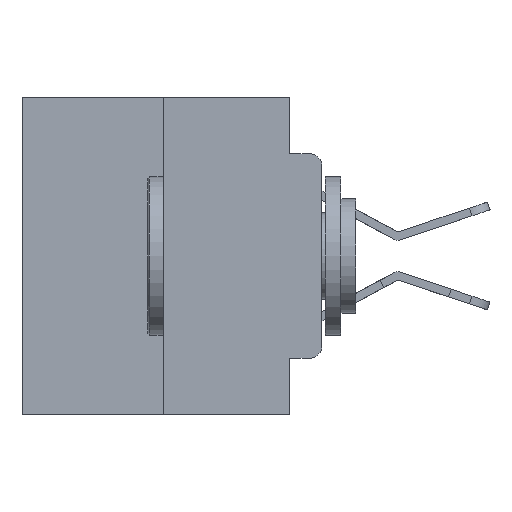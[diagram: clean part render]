
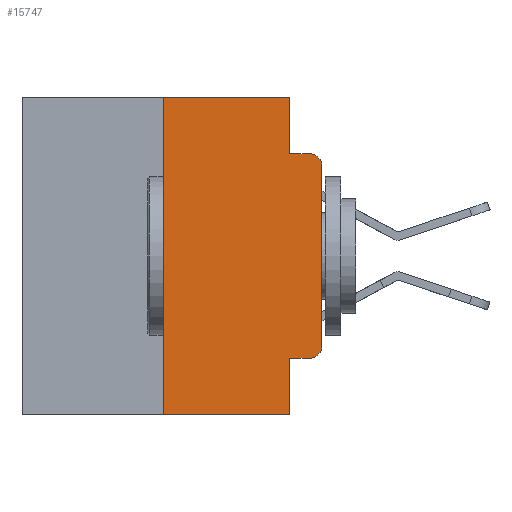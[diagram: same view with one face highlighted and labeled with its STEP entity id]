
A CAD part, left-side view. The second image highlights one B-rep face of the part: STEP entity #15747.
In plain terms, the highlighted planar face has unit normal (-1, 0, 0).
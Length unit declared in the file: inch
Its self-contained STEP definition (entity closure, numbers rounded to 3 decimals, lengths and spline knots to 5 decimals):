
#317 = VECTOR ( 'NONE', #20871, 39.37008 ) ;
#579 = LINE ( 'NONE', #9387, #16527 ) ;
#1281 = CARTESIAN_POINT ( 'NONE',  ( 0., 0.051, -0.5 ) ) ;
#1337 = AXIS2_PLACEMENT_3D ( 'NONE', #26024, #19266, #27897 ) ;
#2168 = CARTESIAN_POINT ( 'NONE',  ( 0., 0.473, 0. ) ) ;
#2622 = EDGE_CURVE ( 'NONE', #16160, #18057, #3386, .T. ) ;
#3017 = LINE ( 'NONE', #12999, #14215 ) ;
#3018 = LINE ( 'NONE', #6494, #4365 ) ;
#3276 = CARTESIAN_POINT ( 'NONE',  ( 0., 0., -0.1085 ) ) ;
#3386 = CIRCLE ( 'NONE', #24783, 0.02 ) ;
#3666 = ORIENTED_EDGE ( 'NONE', *, *, #14848, .F. ) ;
#4170 = DIRECTION ( 'NONE',  ( 0., 0., 1. ) ) ;
#4365 = VECTOR ( 'NONE', #12855, 39.37008 ) ;
#4695 = VERTEX_POINT ( 'NONE', #11826 ) ;
#5046 = DIRECTION ( 'NONE',  ( -1., 0., 0. ) ) ;
#5175 = ORIENTED_EDGE ( 'NONE', *, *, #15756, .F. ) ;
#5534 = ORIENTED_EDGE ( 'NONE', *, *, #21497, .F. ) ;
#5602 = VERTEX_POINT ( 'NONE', #13265 ) ;
#6494 = CARTESIAN_POINT ( 'NONE',  ( 0., 0.051, -0.4115 ) ) ;
#7462 = EDGE_CURVE ( 'NONE', #5602, #18057, #14799, .T. ) ;
#7708 = CARTESIAN_POINT ( 'NONE',  ( 0., 0.25, 0. ) ) ;
#8245 = ORIENTED_EDGE ( 'NONE', *, *, #12480, .T. ) ;
#8300 = VECTOR ( 'NONE', #27988, 39.37008 ) ;
#9171 = CARTESIAN_POINT ( 'NONE',  ( 0., 0.051, -0.0885 ) ) ;
#9387 = CARTESIAN_POINT ( 'NONE',  ( 0., 0.051, 0. ) ) ;
#9990 = CARTESIAN_POINT ( 'NONE',  ( 0., 0.051, 0. ) ) ;
#10444 = FACE_OUTER_BOUND ( 'NONE', #14128, .T. ) ;
#10474 = PLANE ( 'NONE',  #1337 ) ;
#10488 = ORIENTED_EDGE ( 'NONE', *, *, #23070, .T. ) ;
#10975 = CARTESIAN_POINT ( 'NONE',  ( 0., 0.051, 0. ) ) ;
#11575 = DIRECTION ( 'NONE',  ( 0., 0., -1. ) ) ;
#11676 = CARTESIAN_POINT ( 'NONE',  ( 0., 0.02, -0.3915 ) ) ;
#11826 = CARTESIAN_POINT ( 'NONE',  ( 0., 0., -0.3915 ) ) ;
#12281 = CARTESIAN_POINT ( 'NONE',  ( 0., 0., 0. ) ) ;
#12480 = EDGE_CURVE ( 'NONE', #4695, #16160, #27333, .T. ) ;
#12764 = VECTOR ( 'NONE', #26627, 39.37008 ) ;
#12842 = VECTOR ( 'NONE', #21733, 39.37008 ) ;
#12855 = DIRECTION ( 'NONE',  ( 0., -1., 0. ) ) ;
#12999 = CARTESIAN_POINT ( 'NONE',  ( 0., 0.25, 0. ) ) ;
#13265 = CARTESIAN_POINT ( 'NONE',  ( 0., 0.051, -0.0885 ) ) ;
#14128 = EDGE_LOOP ( 'NONE', ( #8245, #16524, #21455, #3666, #5175, #5534, #14448, #25004, #19703, #10488 ) ) ;
#14215 = VECTOR ( 'NONE', #4170, 39.37008 ) ;
#14448 = ORIENTED_EDGE ( 'NONE', *, *, #24112, .T. ) ;
#14799 = LINE ( 'NONE', #9171, #12764 ) ;
#14836 = AXIS2_PLACEMENT_3D ( 'NONE', #11676, #5046, #20652 ) ;
#14848 = EDGE_CURVE ( 'NONE', #26928, #5602, #16633, .T. ) ;
#15747 = ADVANCED_FACE ( 'NONE', ( #10444 ), #10474, .F. ) ;
#15756 = EDGE_CURVE ( 'NONE', #20516, #26928, #20701, .T. ) ;
#16160 = VERTEX_POINT ( 'NONE', #3276 ) ;
#16524 = ORIENTED_EDGE ( 'NONE', *, *, #2622, .T. ) ;
#16527 = VECTOR ( 'NONE', #11575, 39.37008 ) ;
#16633 = LINE ( 'NONE', #9990, #317 ) ;
#16810 = EDGE_CURVE ( 'NONE', #26900, #23281, #579, .T. ) ;
#17879 = CARTESIAN_POINT ( 'NONE',  ( 0., 0.051, -0.4115 ) ) ;
#18057 = VERTEX_POINT ( 'NONE', #27667 ) ;
#18267 = DIRECTION ( 'NONE',  ( -1., 0., 0. ) ) ;
#18940 = CIRCLE ( 'NONE', #14836, 0.02 ) ;
#19266 = DIRECTION ( 'NONE',  ( 1., 0., 0. ) ) ;
#19703 = ORIENTED_EDGE ( 'NONE', *, *, #26131, .T. ) ;
#20065 = DIRECTION ( 'NONE',  ( 0., 0., -1. ) ) ;
#20502 = VECTOR ( 'NONE', #23434, 39.37008 ) ;
#20516 = VERTEX_POINT ( 'NONE', #7708 ) ;
#20652 = DIRECTION ( 'NONE',  ( 0., 0., -1. ) ) ;
#20701 = LINE ( 'NONE', #2168, #12842 ) ;
#20871 = DIRECTION ( 'NONE',  ( 0., 0., -1. ) ) ;
#20997 = VERTEX_POINT ( 'NONE', #21875 ) ;
#21455 = ORIENTED_EDGE ( 'NONE', *, *, #7462, .F. ) ;
#21497 = EDGE_CURVE ( 'NONE', #25730, #20516, #3017, .T. ) ;
#21733 = DIRECTION ( 'NONE',  ( 0., -1., 0. ) ) ;
#21875 = CARTESIAN_POINT ( 'NONE',  ( 0., 0.02, -0.4115 ) ) ;
#22347 = CARTESIAN_POINT ( 'NONE',  ( 0., 0.02, -0.1085 ) ) ;
#23070 = EDGE_CURVE ( 'NONE', #20997, #4695, #18940, .T. ) ;
#23281 = VERTEX_POINT ( 'NONE', #1281 ) ;
#23434 = DIRECTION ( 'NONE',  ( 0., 0., 1. ) ) ;
#24112 = EDGE_CURVE ( 'NONE', #25730, #23281, #28121, .T. ) ;
#24783 = AXIS2_PLACEMENT_3D ( 'NONE', #22347, #18267, #20065 ) ;
#25004 = ORIENTED_EDGE ( 'NONE', *, *, #16810, .F. ) ;
#25730 = VERTEX_POINT ( 'NONE', #26893 ) ;
#25931 = CARTESIAN_POINT ( 'NONE',  ( 0., 0.473, -0.5 ) ) ;
#26024 = CARTESIAN_POINT ( 'NONE',  ( 0., 0.473, 0. ) ) ;
#26131 = EDGE_CURVE ( 'NONE', #26900, #20997, #3018, .T. ) ;
#26627 = DIRECTION ( 'NONE',  ( 0., -1., 0. ) ) ;
#26893 = CARTESIAN_POINT ( 'NONE',  ( 0., 0.25, -0.5 ) ) ;
#26900 = VERTEX_POINT ( 'NONE', #17879 ) ;
#26928 = VERTEX_POINT ( 'NONE', #10975 ) ;
#27333 = LINE ( 'NONE', #12281, #20502 ) ;
#27667 = CARTESIAN_POINT ( 'NONE',  ( 0., 0.02, -0.0885 ) ) ;
#27897 = DIRECTION ( 'NONE',  ( 0., 0., -1. ) ) ;
#27988 = DIRECTION ( 'NONE',  ( 0., -1., 0. ) ) ;
#28121 = LINE ( 'NONE', #25931, #8300 ) ;
